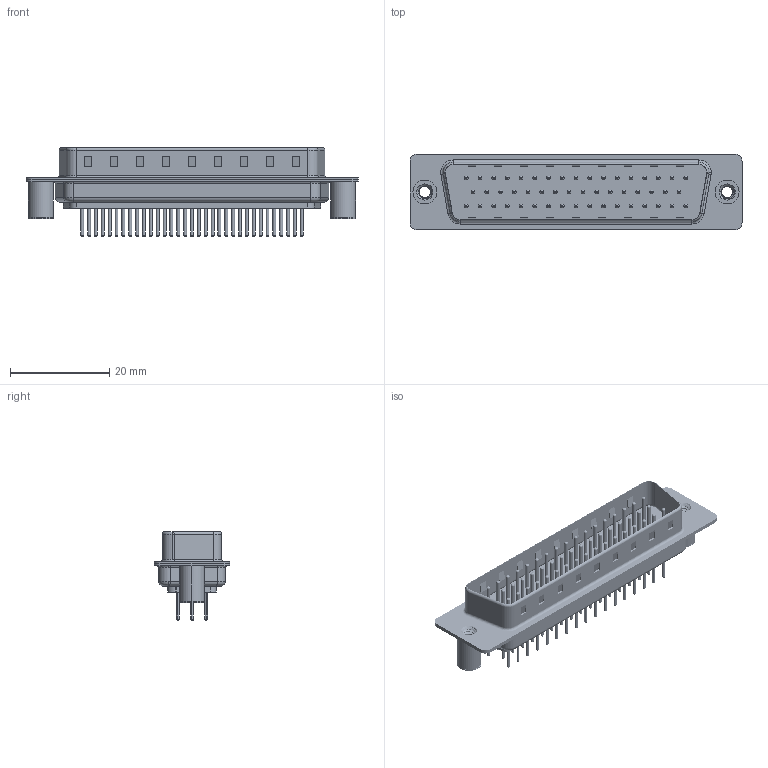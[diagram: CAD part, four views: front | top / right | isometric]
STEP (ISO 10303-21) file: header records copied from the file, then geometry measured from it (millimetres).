
FILE_DESCRIPTION (( 'STEP AP203' ), '1' );
FILE_NAME ('627-M50-320-WN3.STEP', '2020-07-17T18:04:17', ( '' ), ( '' ), 'SwSTEP 2.0', 'SolidWorks 2020', '' );
FILE_SCHEMA (( 'CONFIG_CONTROL_DESIGN' ));
Length unit declared in the file: millimetre
Products named in the file (8): 627M Contact Row 3_20; 627M Contact Row 1_20; 627-M50-320-WN3; 627M Shell Rear_50 Contacts; 627M Contact Row 2_20; 627M Shell Front_50 Contacts; 627M Housing_50 Contacts; 627M 4-40 Threaded Board Spacer
Assembly tree (55 placements, depth 2):
  627-M50-320-WN3
    627M Housing_50 Contacts
    627M Shell Front_50 Contacts
    627M Shell Rear_50 Contacts
    627M Contact Row 1_20  x17
    627M Contact Row 2_20  x16
    627M Contact Row 3_20  x17
    627M 4-40 Threaded Board Spacer  x2
Bounding box: 67 x 15.3 x 17.9 mm (x, y, z)
Volume: 4647.6 mm3; surface area: 10957.4 mm2
Topology: 55 solids, 55 shells, 2296 faces, 4841 edges, 2916 vertices
Faces by surface type: cylinder 865, torus 854, plane 553, cone 18, bspline 6
Entity records: 29899 total; most frequent: CARTESIAN_POINT 6094, DIRECTION 4951, ORIENTED_EDGE 4172, EDGE_CURVE 2086, AXIS2_PLACEMENT_3D 1990, VERTEX_POINT 1335, EDGE_LOOP 1151, CIRCLE 1052
